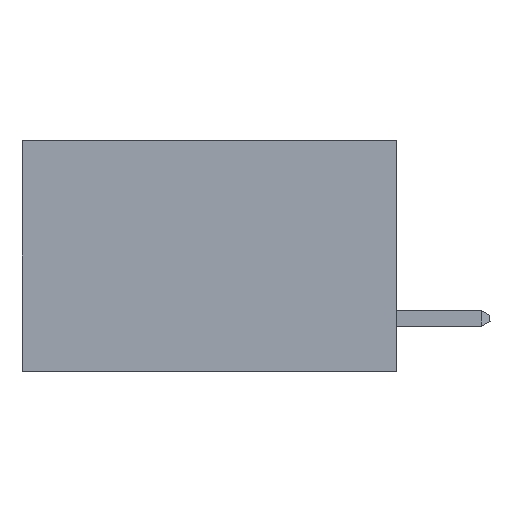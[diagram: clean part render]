
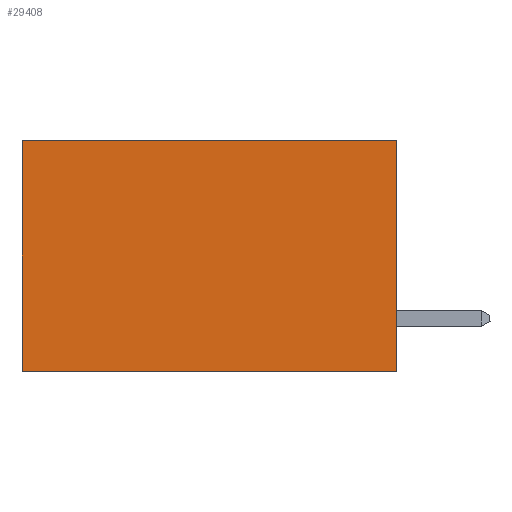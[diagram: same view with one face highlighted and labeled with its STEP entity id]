
A CAD part, left-side view. The second image highlights one B-rep face of the part: STEP entity #29408.
In plain terms, the highlighted planar face has unit normal (-1, 0, 0).
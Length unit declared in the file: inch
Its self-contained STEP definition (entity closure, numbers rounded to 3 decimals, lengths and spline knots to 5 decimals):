
#2411 = VECTOR ( 'NONE', #12361, 39.37008 ) ;
#2591 = EDGE_CURVE ( 'NONE', #3436, #6001, #26391, .T. ) ;
#3436 = VERTEX_POINT ( 'NONE', #9584 ) ;
#6001 = VERTEX_POINT ( 'NONE', #29722 ) ;
#6820 = EDGE_LOOP ( 'NONE', ( #28054, #12758, #13065, #19683 ) ) ;
#7743 = DIRECTION ( 'NONE',  ( 0., 0., -1. ) ) ;
#7967 = LINE ( 'NONE', #16704, #18325 ) ;
#9046 = EDGE_CURVE ( 'NONE', #3436, #26843, #25361, .T. ) ;
#9101 = LINE ( 'NONE', #15618, #25910 ) ;
#9584 = CARTESIAN_POINT ( 'NONE',  ( 0.298, 0., 0. ) ) ;
#12242 = FACE_OUTER_BOUND ( 'NONE', #6820, .T. ) ;
#12361 = DIRECTION ( 'NONE',  ( 0., 1., 0. ) ) ;
#12758 = ORIENTED_EDGE ( 'NONE', *, *, #28533, .F. ) ;
#13065 = ORIENTED_EDGE ( 'NONE', *, *, #2591, .F. ) ;
#13165 = CARTESIAN_POINT ( 'NONE',  ( 0.298, 0., 0. ) ) ;
#14230 = VECTOR ( 'NONE', #24473, 39.37008 ) ;
#15182 = EDGE_CURVE ( 'NONE', #26843, #19226, #7967, .T. ) ;
#15618 = CARTESIAN_POINT ( 'NONE',  ( 0.298, 0., -0.37 ) ) ;
#15973 = DIRECTION ( 'NONE',  ( 1., 0., 0. ) ) ;
#16500 = CARTESIAN_POINT ( 'NONE',  ( 0.298, 0.6, 0. ) ) ;
#16704 = CARTESIAN_POINT ( 'NONE',  ( 0.298, 0.6, 0. ) ) ;
#17543 = CARTESIAN_POINT ( 'NONE',  ( 0.298, 0.6, -0.37 ) ) ;
#17896 = DIRECTION ( 'NONE',  ( 0., 1., 0. ) ) ;
#18325 = VECTOR ( 'NONE', #19305, 39.37008 ) ;
#19226 = VERTEX_POINT ( 'NONE', #17543 ) ;
#19305 = DIRECTION ( 'NONE',  ( 0., 0., -1. ) ) ;
#19683 = ORIENTED_EDGE ( 'NONE', *, *, #9046, .T. ) ;
#23772 = CARTESIAN_POINT ( 'NONE',  ( 0.298, 0., 0. ) ) ;
#24473 = DIRECTION ( 'NONE',  ( 0., 0., -1. ) ) ;
#25361 = LINE ( 'NONE', #23772, #2411 ) ;
#25910 = VECTOR ( 'NONE', #17896, 39.37008 ) ;
#26391 = LINE ( 'NONE', #13165, #14230 ) ;
#26843 = VERTEX_POINT ( 'NONE', #16500 ) ;
#27367 = PLANE ( 'NONE',  #29194 ) ;
#28054 = ORIENTED_EDGE ( 'NONE', *, *, #15182, .T. ) ;
#28533 = EDGE_CURVE ( 'NONE', #6001, #19226, #9101, .T. ) ;
#29194 = AXIS2_PLACEMENT_3D ( 'NONE', #29679, #15973, #7743 ) ;
#29408 = ADVANCED_FACE ( 'NONE', ( #12242 ), #27367, .F. ) ;
#29679 = CARTESIAN_POINT ( 'NONE',  ( 0.298, 0., 0. ) ) ;
#29722 = CARTESIAN_POINT ( 'NONE',  ( 0.298, 0., -0.37 ) ) ;
